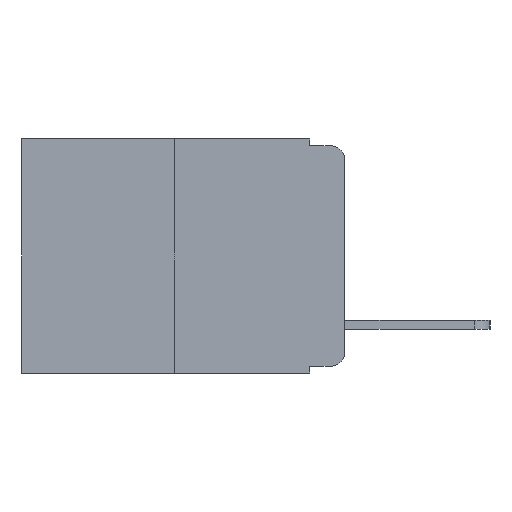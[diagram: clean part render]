
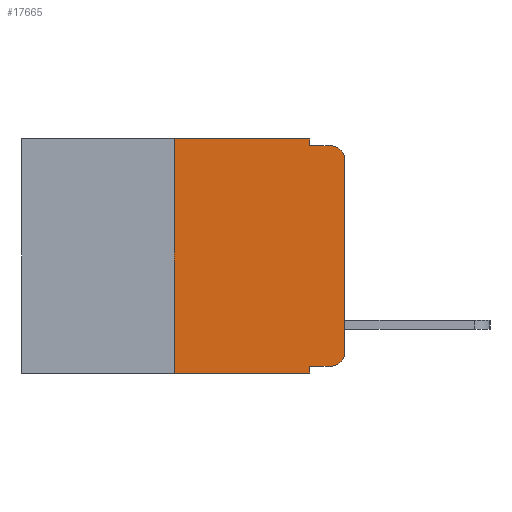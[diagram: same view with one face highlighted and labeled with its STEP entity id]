
A CAD part, left-side view. The second image highlights one B-rep face of the part: STEP entity #17665.
In plain terms, the highlighted planar face has unit normal (-1, 0, 0).
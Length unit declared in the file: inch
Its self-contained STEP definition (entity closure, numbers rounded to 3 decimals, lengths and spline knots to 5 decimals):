
#594 = CARTESIAN_POINT ( 'NONE',  ( 0., 0.051, 0. ) ) ;
#603 = EDGE_CURVE ( 'NONE', #3515, #15791, #17738, .T. ) ;
#987 = VECTOR ( 'NONE', #20573, 39.37008 ) ;
#1352 = DIRECTION ( 'NONE',  ( -1., 0., 0. ) ) ;
#1824 = CARTESIAN_POINT ( 'NONE',  ( 0., 0.25, -0.343 ) ) ;
#2413 = VERTEX_POINT ( 'NONE', #1824 ) ;
#2422 = CARTESIAN_POINT ( 'NONE',  ( 0., 0.051, -0.01 ) ) ;
#2700 = ORIENTED_EDGE ( 'NONE', *, *, #21972, .F. ) ;
#2936 = ORIENTED_EDGE ( 'NONE', *, *, #8386, .T. ) ;
#3167 = EDGE_LOOP ( 'NONE', ( #4297, #5751, #5019, #2700, #19895, #17021, #17518, #3915, #2936, #8704 ) ) ;
#3265 = CARTESIAN_POINT ( 'NONE',  ( 0., 0.473, 0. ) ) ;
#3515 = VERTEX_POINT ( 'NONE', #9714 ) ;
#3891 = LINE ( 'NONE', #594, #8424 ) ;
#3915 = ORIENTED_EDGE ( 'NONE', *, *, #603, .F. ) ;
#3968 = EDGE_CURVE ( 'NONE', #10704, #9686, #20829, .T. ) ;
#4015 = AXIS2_PLACEMENT_3D ( 'NONE', #16968, #13687, #20608 ) ;
#4120 = AXIS2_PLACEMENT_3D ( 'NONE', #11707, #1352, #17151 ) ;
#4153 = VECTOR ( 'NONE', #17477, 39.37008 ) ;
#4297 = ORIENTED_EDGE ( 'NONE', *, *, #7600, .T. ) ;
#4713 = VERTEX_POINT ( 'NONE', #19628 ) ;
#4985 = LINE ( 'NONE', #22307, #987 ) ;
#5019 = ORIENTED_EDGE ( 'NONE', *, *, #8709, .F. ) ;
#5484 = CARTESIAN_POINT ( 'NONE',  ( 0., 0.25, 0. ) ) ;
#5488 = DIRECTION ( 'NONE',  ( 0., 0., -1. ) ) ;
#5663 = FACE_OUTER_BOUND ( 'NONE', #3167, .T. ) ;
#5751 = ORIENTED_EDGE ( 'NONE', *, *, #3968, .T. ) ;
#6362 = AXIS2_PLACEMENT_3D ( 'NONE', #14419, #12496, #21241 ) ;
#7084 = CARTESIAN_POINT ( 'NONE',  ( 0., 0.051, 0. ) ) ;
#7458 = EDGE_CURVE ( 'NONE', #2413, #15791, #4985, .T. ) ;
#7600 = EDGE_CURVE ( 'NONE', #4713, #10704, #19439, .T. ) ;
#8386 = EDGE_CURVE ( 'NONE', #3515, #12695, #13708, .T. ) ;
#8424 = VECTOR ( 'NONE', #5488, 39.37008 ) ;
#8457 = CARTESIAN_POINT ( 'NONE',  ( 0., 0.051, -0.01 ) ) ;
#8704 = ORIENTED_EDGE ( 'NONE', *, *, #19454, .T. ) ;
#8709 = EDGE_CURVE ( 'NONE', #9911, #9686, #13578, .T. ) ;
#8862 = CARTESIAN_POINT ( 'NONE',  ( 0., 0.25, 0. ) ) ;
#9232 = DIRECTION ( 'NONE',  ( 0., 0., -1. ) ) ;
#9686 = VERTEX_POINT ( 'NONE', #18932 ) ;
#9714 = CARTESIAN_POINT ( 'NONE',  ( 0., 0.051, -0.333 ) ) ;
#9911 = VERTEX_POINT ( 'NONE', #2422 ) ;
#10704 = VERTEX_POINT ( 'NONE', #20740 ) ;
#11505 = VECTOR ( 'NONE', #9232, 39.37008 ) ;
#11707 = CARTESIAN_POINT ( 'NONE',  ( 0., 0.02, -0.03 ) ) ;
#11937 = VECTOR ( 'NONE', #22224, 39.37008 ) ;
#12496 = DIRECTION ( 'NONE',  ( 1., 0., 0. ) ) ;
#12695 = VERTEX_POINT ( 'NONE', #20582 ) ;
#13246 = VERTEX_POINT ( 'NONE', #8862 ) ;
#13334 = VECTOR ( 'NONE', #16034, 39.37008 ) ;
#13578 = LINE ( 'NONE', #8457, #11937 ) ;
#13687 = DIRECTION ( 'NONE',  ( -1., 0., 0. ) ) ;
#13708 = LINE ( 'NONE', #16892, #22476 ) ;
#14382 = EDGE_CURVE ( 'NONE', #2413, #13246, #21062, .T. ) ;
#14419 = CARTESIAN_POINT ( 'NONE',  ( 0., 0.473, 0. ) ) ;
#14554 = CIRCLE ( 'NONE', #4015, 0.02 ) ;
#14597 = DIRECTION ( 'NONE',  ( 0., 0., 1. ) ) ;
#15791 = VERTEX_POINT ( 'NONE', #19099 ) ;
#15807 = LINE ( 'NONE', #3265, #4153 ) ;
#16034 = DIRECTION ( 'NONE',  ( 0., 0., 1. ) ) ;
#16513 = CARTESIAN_POINT ( 'NONE',  ( 0., 0.051, 0. ) ) ;
#16892 = CARTESIAN_POINT ( 'NONE',  ( 0., 0.051, -0.333 ) ) ;
#16968 = CARTESIAN_POINT ( 'NONE',  ( 0., 0.02, -0.313 ) ) ;
#17021 = ORIENTED_EDGE ( 'NONE', *, *, #14382, .F. ) ;
#17151 = DIRECTION ( 'NONE',  ( 0., 0., -1. ) ) ;
#17477 = DIRECTION ( 'NONE',  ( 0., -1., 0. ) ) ;
#17485 = EDGE_CURVE ( 'NONE', #13246, #19687, #15807, .T. ) ;
#17518 = ORIENTED_EDGE ( 'NONE', *, *, #7458, .T. ) ;
#17665 = ADVANCED_FACE ( 'NONE', ( #5663 ), #21579, .F. ) ;
#17738 = LINE ( 'NONE', #7084, #11505 ) ;
#18705 = DIRECTION ( 'NONE',  ( 0., -1., 0. ) ) ;
#18932 = CARTESIAN_POINT ( 'NONE',  ( 0., 0.02, -0.01 ) ) ;
#19099 = CARTESIAN_POINT ( 'NONE',  ( 0., 0.051, -0.343 ) ) ;
#19439 = LINE ( 'NONE', #21019, #13334 ) ;
#19454 = EDGE_CURVE ( 'NONE', #12695, #4713, #14554, .T. ) ;
#19628 = CARTESIAN_POINT ( 'NONE',  ( 0., 0., -0.313 ) ) ;
#19687 = VERTEX_POINT ( 'NONE', #16513 ) ;
#19895 = ORIENTED_EDGE ( 'NONE', *, *, #17485, .F. ) ;
#20573 = DIRECTION ( 'NONE',  ( 0., -1., 0. ) ) ;
#20582 = CARTESIAN_POINT ( 'NONE',  ( 0., 0.02, -0.333 ) ) ;
#20608 = DIRECTION ( 'NONE',  ( 0., 0., -1. ) ) ;
#20740 = CARTESIAN_POINT ( 'NONE',  ( 0., 0., -0.03 ) ) ;
#20829 = CIRCLE ( 'NONE', #4120, 0.02 ) ;
#21019 = CARTESIAN_POINT ( 'NONE',  ( 0., 0., 0. ) ) ;
#21062 = LINE ( 'NONE', #5484, #21530 ) ;
#21241 = DIRECTION ( 'NONE',  ( 0., 0., -1. ) ) ;
#21530 = VECTOR ( 'NONE', #14597, 39.37008 ) ;
#21579 = PLANE ( 'NONE',  #6362 ) ;
#21972 = EDGE_CURVE ( 'NONE', #19687, #9911, #3891, .T. ) ;
#22224 = DIRECTION ( 'NONE',  ( 0., -1., 0. ) ) ;
#22307 = CARTESIAN_POINT ( 'NONE',  ( 0., 0.473, -0.343 ) ) ;
#22476 = VECTOR ( 'NONE', #18705, 39.37008 ) ;
